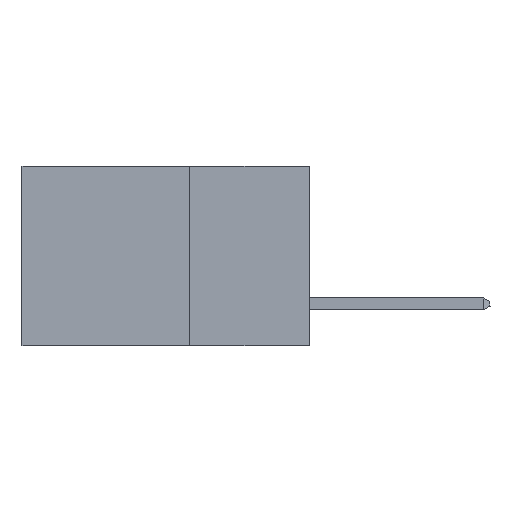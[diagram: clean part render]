
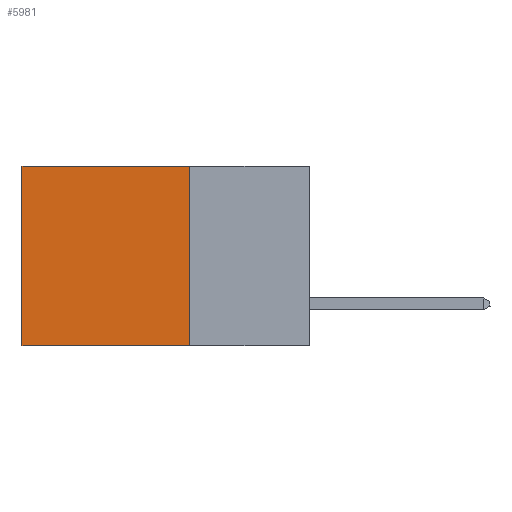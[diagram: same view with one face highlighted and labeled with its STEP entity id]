
A CAD part, left-side view. The second image highlights one B-rep face of the part: STEP entity #5981.
In plain terms, the highlighted planar face has unit normal (-1, 0, 0).
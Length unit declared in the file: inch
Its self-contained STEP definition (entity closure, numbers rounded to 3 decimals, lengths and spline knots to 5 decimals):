
#60 = LINE ( 'NONE', #10131, #1661 ) ;
#181 = CARTESIAN_POINT ( 'NONE',  ( 0.2875, 0.25, -0.375 ) ) ;
#924 = VECTOR ( 'NONE', #6063, 39.37008 ) ;
#1035 = FACE_OUTER_BOUND ( 'NONE', #8135, .T. ) ;
#1060 = CARTESIAN_POINT ( 'NONE',  ( 0.2875, 0.25, 0. ) ) ;
#1661 = VECTOR ( 'NONE', #5073, 39.37008 ) ;
#1825 = DIRECTION ( 'NONE',  ( 0., 1., 0. ) ) ;
#2523 = VERTEX_POINT ( 'NONE', #1060 ) ;
#3770 = CARTESIAN_POINT ( 'NONE',  ( 0.2875, 0.25, 0. ) ) ;
#3973 = CARTESIAN_POINT ( 'NONE',  ( 0.2875, 0.25, -0.375 ) ) ;
#4063 = CARTESIAN_POINT ( 'NONE',  ( 0.2875, 0.6, -0.375 ) ) ;
#4402 = AXIS2_PLACEMENT_3D ( 'NONE', #3973, #9977, #12976 ) ;
#5073 = DIRECTION ( 'NONE',  ( 0., 0., -1. ) ) ;
#5205 = CARTESIAN_POINT ( 'NONE',  ( 0.2875, 0.6, -0.375 ) ) ;
#5765 = DIRECTION ( 'NONE',  ( 0., 1., 0. ) ) ;
#5981 = ADVANCED_FACE ( 'NONE', ( #1035 ), #11172, .F. ) ;
#6063 = DIRECTION ( 'NONE',  ( 0., 0., -1. ) ) ;
#6498 = VECTOR ( 'NONE', #5765, 39.37008 ) ;
#6891 = VECTOR ( 'NONE', #1825, 39.37008 ) ;
#6973 = LINE ( 'NONE', #3770, #6891 ) ;
#6982 = VERTEX_POINT ( 'NONE', #181 ) ;
#7135 = ORIENTED_EDGE ( 'NONE', *, *, #9410, .F. ) ;
#7609 = EDGE_CURVE ( 'NONE', #2523, #11917, #6973, .T. ) ;
#7690 = ORIENTED_EDGE ( 'NONE', *, *, #9911, .F. ) ;
#8135 = EDGE_LOOP ( 'NONE', ( #12435, #7135, #7690, #8601 ) ) ;
#8601 = ORIENTED_EDGE ( 'NONE', *, *, #7609, .T. ) ;
#8656 = EDGE_CURVE ( 'NONE', #11917, #12117, #10127, .T. ) ;
#9410 = EDGE_CURVE ( 'NONE', #6982, #12117, #9957, .T. ) ;
#9911 = EDGE_CURVE ( 'NONE', #2523, #6982, #60, .T. ) ;
#9957 = LINE ( 'NONE', #12021, #6498 ) ;
#9977 = DIRECTION ( 'NONE',  ( 1., 0., 0. ) ) ;
#10127 = LINE ( 'NONE', #4063, #924 ) ;
#10131 = CARTESIAN_POINT ( 'NONE',  ( 0.2875, 0.25, -0.375 ) ) ;
#10948 = CARTESIAN_POINT ( 'NONE',  ( 0.2875, 0.6, 0. ) ) ;
#11172 = PLANE ( 'NONE',  #4402 ) ;
#11917 = VERTEX_POINT ( 'NONE', #10948 ) ;
#12021 = CARTESIAN_POINT ( 'NONE',  ( 0.2875, 0.25, -0.375 ) ) ;
#12117 = VERTEX_POINT ( 'NONE', #5205 ) ;
#12435 = ORIENTED_EDGE ( 'NONE', *, *, #8656, .T. ) ;
#12976 = DIRECTION ( 'NONE',  ( 0., 0., -1. ) ) ;
